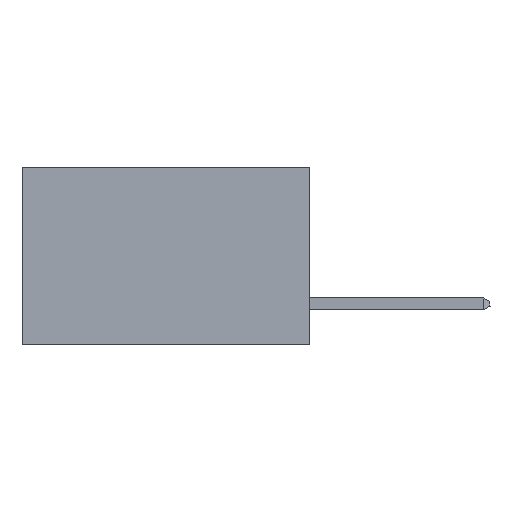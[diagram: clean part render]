
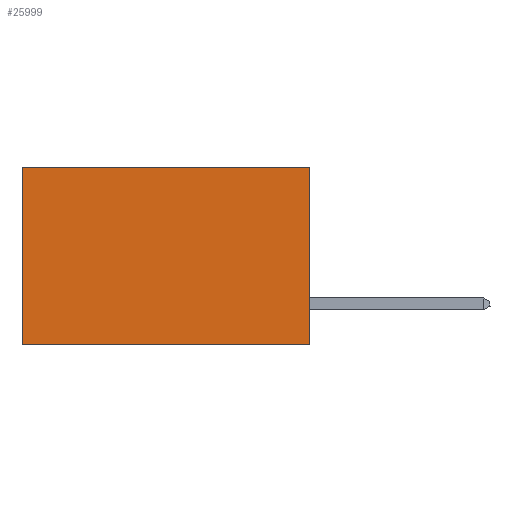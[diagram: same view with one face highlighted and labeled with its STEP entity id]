
A CAD part, left-side view. The second image highlights one B-rep face of the part: STEP entity #25999.
In plain terms, the highlighted planar face has unit normal (-1, 0, 0).
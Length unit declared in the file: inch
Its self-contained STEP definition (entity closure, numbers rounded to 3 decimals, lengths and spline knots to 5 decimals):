
#16 = VECTOR ( 'NONE', #35570, 39.37008 ) ;
#723 = DIRECTION ( 'NONE',  ( 0., 0., -1. ) ) ;
#763 = VERTEX_POINT ( 'NONE', #37408 ) ;
#1054 = LINE ( 'NONE', #22188, #16 ) ;
#2052 = VECTOR ( 'NONE', #723, 39.37008 ) ;
#2241 = EDGE_CURVE ( 'NONE', #37301, #20472, #36373, .T. ) ;
#2664 = ORIENTED_EDGE ( 'NONE', *, *, #2241, .T. ) ;
#3915 = CARTESIAN_POINT ( 'NONE',  ( 0.2875, 0., 0. ) ) ;
#4125 = LINE ( 'NONE', #13824, #21063 ) ;
#7541 = AXIS2_PLACEMENT_3D ( 'NONE', #28425, #12309, #31718 ) ;
#11773 = ORIENTED_EDGE ( 'NONE', *, *, #35407, .F. ) ;
#12309 = DIRECTION ( 'NONE',  ( 1., 0., 0. ) ) ;
#13824 = CARTESIAN_POINT ( 'NONE',  ( 0.2875, 0., 0. ) ) ;
#16660 = CARTESIAN_POINT ( 'NONE',  ( 0.2875, 0.6, 0. ) ) ;
#17377 = CARTESIAN_POINT ( 'NONE',  ( 0.2875, 0., 0. ) ) ;
#17952 = DIRECTION ( 'NONE',  ( 0., 0., -1. ) ) ;
#20472 = VERTEX_POINT ( 'NONE', #21742 ) ;
#21063 = VECTOR ( 'NONE', #39527, 39.37008 ) ;
#21742 = CARTESIAN_POINT ( 'NONE',  ( 0.2875, 0.6, -0.37 ) ) ;
#22188 = CARTESIAN_POINT ( 'NONE',  ( 0.2875, 0., -0.37 ) ) ;
#24115 = LINE ( 'NONE', #3915, #2052 ) ;
#24160 = ORIENTED_EDGE ( 'NONE', *, *, #41664, .F. ) ;
#25999 = ADVANCED_FACE ( 'NONE', ( #33873 ), #35149, .F. ) ;
#28425 = CARTESIAN_POINT ( 'NONE',  ( 0.2875, 0., 0. ) ) ;
#28670 = ORIENTED_EDGE ( 'NONE', *, *, #41652, .T. ) ;
#31718 = DIRECTION ( 'NONE',  ( 0., 0., -1. ) ) ;
#33873 = FACE_OUTER_BOUND ( 'NONE', #34585, .T. ) ;
#34382 = CARTESIAN_POINT ( 'NONE',  ( 0.2875, 0.6, 0. ) ) ;
#34585 = EDGE_LOOP ( 'NONE', ( #2664, #11773, #24160, #28670 ) ) ;
#35149 = PLANE ( 'NONE',  #7541 ) ;
#35407 = EDGE_CURVE ( 'NONE', #763, #20472, #1054, .T. ) ;
#35570 = DIRECTION ( 'NONE',  ( 0., 1., 0. ) ) ;
#36373 = LINE ( 'NONE', #34382, #40473 ) ;
#37301 = VERTEX_POINT ( 'NONE', #16660 ) ;
#37408 = CARTESIAN_POINT ( 'NONE',  ( 0.2875, 0., -0.37 ) ) ;
#37540 = VERTEX_POINT ( 'NONE', #17377 ) ;
#39527 = DIRECTION ( 'NONE',  ( 0., 1., 0. ) ) ;
#40473 = VECTOR ( 'NONE', #17952, 39.37008 ) ;
#41652 = EDGE_CURVE ( 'NONE', #37540, #37301, #4125, .T. ) ;
#41664 = EDGE_CURVE ( 'NONE', #37540, #763, #24115, .T. ) ;
